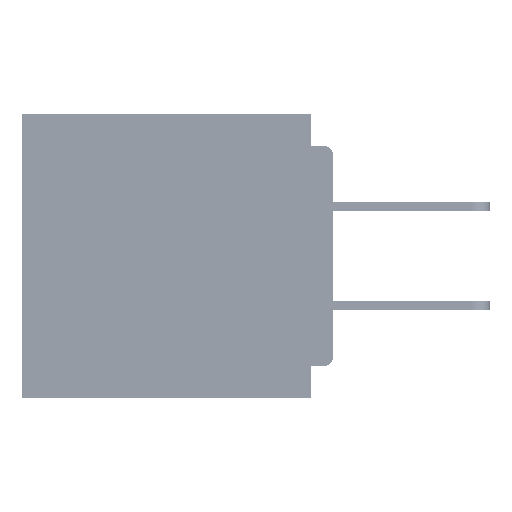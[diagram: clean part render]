
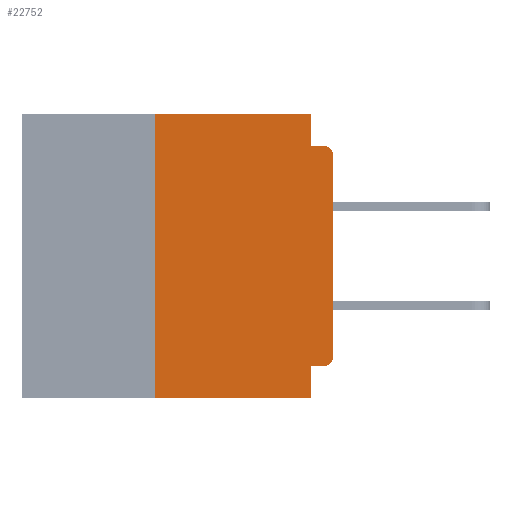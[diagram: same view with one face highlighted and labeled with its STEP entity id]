
A CAD part, left-side view. The second image highlights one B-rep face of the part: STEP entity #22752.
In plain terms, the highlighted planar face has unit normal (-1, 0, 0).
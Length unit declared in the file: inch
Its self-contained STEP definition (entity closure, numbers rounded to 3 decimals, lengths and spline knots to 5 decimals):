
#186 = AXIS2_PLACEMENT_3D ( 'NONE', #65213, #35159, #4931 ) ;
#676 = ORIENTED_EDGE ( 'NONE', *, *, #8338, .T. ) ;
#728 = EDGE_CURVE ( 'NONE', #56220, #21599, #11682, .T. ) ;
#3017 = CARTESIAN_POINT ( 'NONE',  ( 0., 0.031, -0.355 ) ) ;
#3204 = VERTEX_POINT ( 'NONE', #6509 ) ;
#3257 = CARTESIAN_POINT ( 'NONE',  ( 0., 0.25, -0.4 ) ) ;
#3681 = DIRECTION ( 'NONE',  ( 0., -1., 0. ) ) ;
#4154 = CARTESIAN_POINT ( 'NONE',  ( 0., 0.031, -0.4 ) ) ;
#4931 = DIRECTION ( 'NONE',  ( 0., 0., -1. ) ) ;
#5050 = CARTESIAN_POINT ( 'NONE',  ( 0., 0., 0. ) ) ;
#5924 = AXIS2_PLACEMENT_3D ( 'NONE', #49296, #29371, #64482 ) ;
#6509 = CARTESIAN_POINT ( 'NONE',  ( 0., 0.25, -0.4 ) ) ;
#7103 = EDGE_CURVE ( 'NONE', #51268, #56220, #22631, .T. ) ;
#8326 = CIRCLE ( 'NONE', #9394, 0.015 ) ;
#8334 = CARTESIAN_POINT ( 'NONE',  ( 0., 0.25, 0. ) ) ;
#8338 = EDGE_CURVE ( 'NONE', #3204, #63517, #64069, .T. ) ;
#9394 = AXIS2_PLACEMENT_3D ( 'NONE', #12783, #47928, #17863 ) ;
#10305 = PLANE ( 'NONE',  #5924 ) ;
#11682 = LINE ( 'NONE', #61704, #36922 ) ;
#11757 = ORIENTED_EDGE ( 'NONE', *, *, #20175, .T. ) ;
#12783 = CARTESIAN_POINT ( 'NONE',  ( 0., 0.015, -0.06 ) ) ;
#14858 = VERTEX_POINT ( 'NONE', #31322 ) ;
#16594 = LINE ( 'NONE', #5050, #43334 ) ;
#16620 = VERTEX_POINT ( 'NONE', #45814 ) ;
#17863 = DIRECTION ( 'NONE',  ( 0., 0., -1. ) ) ;
#18545 = LINE ( 'NONE', #52277, #43683 ) ;
#18647 = EDGE_CURVE ( 'NONE', #26816, #63517, #61530, .T. ) ;
#19690 = ORIENTED_EDGE ( 'NONE', *, *, #33529, .F. ) ;
#20175 = EDGE_CURVE ( 'NONE', #40284, #14858, #16594, .T. ) ;
#20516 = ORIENTED_EDGE ( 'NONE', *, *, #49778, .F. ) ;
#21599 = VERTEX_POINT ( 'NONE', #41690 ) ;
#22351 = CARTESIAN_POINT ( 'NONE',  ( 0., 0., -0.045 ) ) ;
#22631 = LINE ( 'NONE', #38400, #46170 ) ;
#22752 = ADVANCED_FACE ( 'NONE', ( #35932 ), #10305, .F. ) ;
#25078 = EDGE_CURVE ( 'NONE', #3204, #51268, #38797, .T. ) ;
#25535 = CARTESIAN_POINT ( 'NONE',  ( 0., 0., -0.34 ) ) ;
#26816 = VERTEX_POINT ( 'NONE', #3017 ) ;
#26840 = ORIENTED_EDGE ( 'NONE', *, *, #36665, .T. ) ;
#28684 = VECTOR ( 'NONE', #32453, 39.37008 ) ;
#28862 = CARTESIAN_POINT ( 'NONE',  ( 0., 0.437, -0.4 ) ) ;
#29371 = DIRECTION ( 'NONE',  ( 1., 0., 0. ) ) ;
#30267 = LINE ( 'NONE', #22351, #28684 ) ;
#31322 = CARTESIAN_POINT ( 'NONE',  ( 0., 0., -0.06 ) ) ;
#32126 = CARTESIAN_POINT ( 'NONE',  ( 0., 0.031, -0.4 ) ) ;
#32453 = DIRECTION ( 'NONE',  ( 0., -1., 0. ) ) ;
#33529 = EDGE_CURVE ( 'NONE', #21599, #57736, #30267, .T. ) ;
#34648 = ORIENTED_EDGE ( 'NONE', *, *, #728, .F. ) ;
#35159 = DIRECTION ( 'NONE',  ( -1., 0., 0. ) ) ;
#35281 = DIRECTION ( 'NONE',  ( 0., 0., 1. ) ) ;
#35932 = FACE_OUTER_BOUND ( 'NONE', #45202, .T. ) ;
#36665 = EDGE_CURVE ( 'NONE', #16620, #40284, #52340, .T. ) ;
#36922 = VECTOR ( 'NONE', #63069, 39.37008 ) ;
#37262 = VECTOR ( 'NONE', #58492, 39.37008 ) ;
#38400 = CARTESIAN_POINT ( 'NONE',  ( 0., 0.437, 0. ) ) ;
#38797 = LINE ( 'NONE', #3257, #37262 ) ;
#40284 = VERTEX_POINT ( 'NONE', #25535 ) ;
#41690 = CARTESIAN_POINT ( 'NONE',  ( 0., 0.031, -0.045 ) ) ;
#43334 = VECTOR ( 'NONE', #35281, 39.37008 ) ;
#43423 = DIRECTION ( 'NONE',  ( 0., -1., 0. ) ) ;
#43683 = VECTOR ( 'NONE', #57333, 39.37008 ) ;
#45202 = EDGE_LOOP ( 'NONE', ( #11757, #65238, #19690, #34648, #47981, #51118, #676, #45655, #20516, #26840 ) ) ;
#45655 = ORIENTED_EDGE ( 'NONE', *, *, #18647, .F. ) ;
#45814 = CARTESIAN_POINT ( 'NONE',  ( 0., 0.015, -0.355 ) ) ;
#46170 = VECTOR ( 'NONE', #43423, 39.37008 ) ;
#46582 = VECTOR ( 'NONE', #59610, 39.37008 ) ;
#47928 = DIRECTION ( 'NONE',  ( -1., 0., 0. ) ) ;
#47981 = ORIENTED_EDGE ( 'NONE', *, *, #7103, .F. ) ;
#49089 = VECTOR ( 'NONE', #3681, 39.37008 ) ;
#49296 = CARTESIAN_POINT ( 'NONE',  ( 0., 0.437, 0. ) ) ;
#49308 = EDGE_CURVE ( 'NONE', #14858, #57736, #8326, .T. ) ;
#49778 = EDGE_CURVE ( 'NONE', #16620, #26816, #18545, .T. ) ;
#51118 = ORIENTED_EDGE ( 'NONE', *, *, #25078, .F. ) ;
#51268 = VERTEX_POINT ( 'NONE', #8334 ) ;
#52277 = CARTESIAN_POINT ( 'NONE',  ( 0., 0., -0.355 ) ) ;
#52340 = CIRCLE ( 'NONE', #186, 0.015 ) ;
#53560 = CARTESIAN_POINT ( 'NONE',  ( 0., 0.031, 0. ) ) ;
#56220 = VERTEX_POINT ( 'NONE', #53560 ) ;
#57333 = DIRECTION ( 'NONE',  ( 0., 1., 0. ) ) ;
#57736 = VERTEX_POINT ( 'NONE', #60436 ) ;
#58492 = DIRECTION ( 'NONE',  ( 0., 0., 1. ) ) ;
#59610 = DIRECTION ( 'NONE',  ( 0., 0., -1. ) ) ;
#60436 = CARTESIAN_POINT ( 'NONE',  ( 0., 0.015, -0.045 ) ) ;
#61530 = LINE ( 'NONE', #4154, #46582 ) ;
#61704 = CARTESIAN_POINT ( 'NONE',  ( 0., 0.031, 0. ) ) ;
#63069 = DIRECTION ( 'NONE',  ( 0., 0., -1. ) ) ;
#63517 = VERTEX_POINT ( 'NONE', #32126 ) ;
#64069 = LINE ( 'NONE', #28862, #49089 ) ;
#64482 = DIRECTION ( 'NONE',  ( 0., 0., -1. ) ) ;
#65213 = CARTESIAN_POINT ( 'NONE',  ( 0., 0.015, -0.34 ) ) ;
#65238 = ORIENTED_EDGE ( 'NONE', *, *, #49308, .T. ) ;
